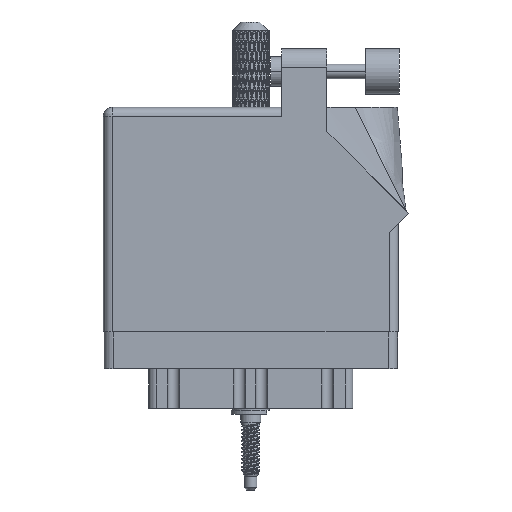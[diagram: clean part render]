
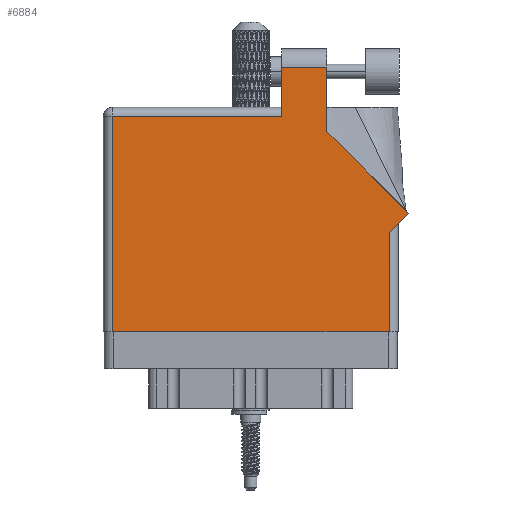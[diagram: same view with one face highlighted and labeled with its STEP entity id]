
A CAD part, front view. The second image highlights one B-rep face of the part: STEP entity #6884.
In plain terms, the highlighted face is planar.
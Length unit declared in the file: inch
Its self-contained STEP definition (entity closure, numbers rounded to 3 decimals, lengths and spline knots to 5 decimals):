
#949 = CARTESIAN_POINT ( 'NONE',  ( 0.062, 0., 0. ) ) ;
#1430 = EDGE_CURVE ( 'NONE', #60707, #52379, #79435, .T. ) ;
#3722 = CARTESIAN_POINT ( 'NONE',  ( 2.08071, 0.80771, 0. ) ) ;
#5582 = CARTESIAN_POINT ( 'NONE',  ( 0., 0., 0. ) ) ;
#5688 = CARTESIAN_POINT ( 'NONE',  ( 1.524, 1.36442, 0. ) ) ;
#5723 = AXIS2_PLACEMENT_3D ( 'NONE', #87404, #56387, #63982 ) ;
#6884 = ADVANCED_FACE ( 'NONE', ( #31912 ), #40078, .F. ) ;
#7382 = DIRECTION ( 'NONE',  ( 0., -1., 0. ) ) ;
#10091 = ORIENTED_EDGE ( 'NONE', *, *, #85054, .T. ) ;
#10898 = LINE ( 'NONE', #3722, #41734 ) ;
#12063 = VERTEX_POINT ( 'NONE', #30886 ) ;
#12244 = DIRECTION ( 'NONE',  ( 1., 0., 0. ) ) ;
#13544 = LINE ( 'NONE', #60405, #100520 ) ;
#14461 = ORIENTED_EDGE ( 'NONE', *, *, #82207, .T. ) ;
#20803 = VECTOR ( 'NONE', #29910, 39.37008 ) ;
#20891 = LINE ( 'NONE', #5582, #59464 ) ;
#21790 = CARTESIAN_POINT ( 'NONE',  ( 2.08071, 0.80771, 0. ) ) ;
#24145 = LINE ( 'NONE', #55262, #75376 ) ;
#25974 = ORIENTED_EDGE ( 'NONE', *, *, #1430, .T. ) ;
#26734 = EDGE_CURVE ( 'NONE', #92078, #84409, #20891, .T. ) ;
#26989 = VECTOR ( 'NONE', #35294, 39.37008 ) ;
#28193 = VERTEX_POINT ( 'NONE', #21790 ) ;
#29910 = DIRECTION ( 'NONE',  ( -1., 0., 0. ) ) ;
#30071 = ORIENTED_EDGE ( 'NONE', *, *, #71883, .T. ) ;
#30886 = CARTESIAN_POINT ( 'NONE',  ( 0.062, 1.468, 0. ) ) ;
#31912 = FACE_OUTER_BOUND ( 'NONE', #76062, .T. ) ;
#33197 = DIRECTION ( 'NONE',  ( 0., 1., 0. ) ) ;
#34224 = CARTESIAN_POINT ( 'NONE',  ( 1.948, 0.737, 0. ) ) ;
#35294 = DIRECTION ( 'NONE',  ( 0.707, 0.707, 0. ) ) ;
#35724 = VECTOR ( 'NONE', #71814, 39.37008 ) ;
#36258 = CARTESIAN_POINT ( 'NONE',  ( 1.948, 0.675, 0. ) ) ;
#40078 = PLANE ( 'NONE',  #5723 ) ;
#41734 = VECTOR ( 'NONE', #73545, 39.37008 ) ;
#41777 = VERTEX_POINT ( 'NONE', #36258 ) ;
#44796 = EDGE_CURVE ( 'NONE', #84409, #41777, #56184, .T. ) ;
#44884 = CARTESIAN_POINT ( 'NONE',  ( 1.524, 1.36442, 0. ) ) ;
#44900 = EDGE_CURVE ( 'NONE', #85499, #60707, #53092, .T. ) ;
#45805 = CARTESIAN_POINT ( 'NONE',  ( 1.217, 1.805, 0. ) ) ;
#50606 = LINE ( 'NONE', #88234, #26989 ) ;
#52379 = VERTEX_POINT ( 'NONE', #45805 ) ;
#52908 = CARTESIAN_POINT ( 'NONE',  ( 0., 1.468, 0. ) ) ;
#53092 = LINE ( 'NONE', #5688, #96048 ) ;
#53731 = VERTEX_POINT ( 'NONE', #63186 ) ;
#55262 = CARTESIAN_POINT ( 'NONE',  ( 1.217, 1.53, 0. ) ) ;
#55530 = CARTESIAN_POINT ( 'NONE',  ( 1.217, 1.805, 0. ) ) ;
#56184 = LINE ( 'NONE', #34224, #81451 ) ;
#56387 = DIRECTION ( 'NONE',  ( 0., 0., -1. ) ) ;
#56633 = CARTESIAN_POINT ( 'NONE',  ( 1.524, 1.805, 0. ) ) ;
#57830 = ORIENTED_EDGE ( 'NONE', *, *, #44796, .T. ) ;
#58045 = LINE ( 'NONE', #52908, #20803 ) ;
#58508 = CARTESIAN_POINT ( 'NONE',  ( 1.948, 0., 0. ) ) ;
#59464 = VECTOR ( 'NONE', #12244, 39.37008 ) ;
#60405 = CARTESIAN_POINT ( 'NONE',  ( 0.062, 0., 0. ) ) ;
#60707 = VERTEX_POINT ( 'NONE', #56633 ) ;
#63186 = CARTESIAN_POINT ( 'NONE',  ( 1.217, 1.468, 0. ) ) ;
#63982 = DIRECTION ( 'NONE',  ( -1., 0., 0. ) ) ;
#71814 = DIRECTION ( 'NONE',  ( -1., 0., 0. ) ) ;
#71883 = EDGE_CURVE ( 'NONE', #12063, #92078, #13544, .T. ) ;
#73545 = DIRECTION ( 'NONE',  ( -0.707, 0.707, 0. ) ) ;
#75376 = VECTOR ( 'NONE', #7382, 39.37008 ) ;
#76062 = EDGE_LOOP ( 'NONE', ( #97641, #25974, #10091, #14461, #30071, #88862, #57830, #99270, #81991 ) ) ;
#79303 = EDGE_CURVE ( 'NONE', #28193, #85499, #10898, .T. ) ;
#79435 = LINE ( 'NONE', #55530, #35724 ) ;
#81451 = VECTOR ( 'NONE', #33197, 39.37008 ) ;
#81991 = ORIENTED_EDGE ( 'NONE', *, *, #79303, .T. ) ;
#82207 = EDGE_CURVE ( 'NONE', #53731, #12063, #58045, .T. ) ;
#84110 = DIRECTION ( 'NONE',  ( 0., 1., 0. ) ) ;
#84409 = VERTEX_POINT ( 'NONE', #58508 ) ;
#85054 = EDGE_CURVE ( 'NONE', #52379, #53731, #24145, .T. ) ;
#85499 = VERTEX_POINT ( 'NONE', #44884 ) ;
#87404 = CARTESIAN_POINT ( 'NONE',  ( 0., 1.53, 0. ) ) ;
#88234 = CARTESIAN_POINT ( 'NONE',  ( 2.01, 0.737, 0. ) ) ;
#88862 = ORIENTED_EDGE ( 'NONE', *, *, #26734, .T. ) ;
#92078 = VERTEX_POINT ( 'NONE', #949 ) ;
#96048 = VECTOR ( 'NONE', #84110, 39.37008 ) ;
#96607 = EDGE_CURVE ( 'NONE', #41777, #28193, #50606, .T. ) ;
#97080 = DIRECTION ( 'NONE',  ( 0., -1., 0. ) ) ;
#97641 = ORIENTED_EDGE ( 'NONE', *, *, #44900, .T. ) ;
#99270 = ORIENTED_EDGE ( 'NONE', *, *, #96607, .T. ) ;
#100520 = VECTOR ( 'NONE', #97080, 39.37008 ) ;
